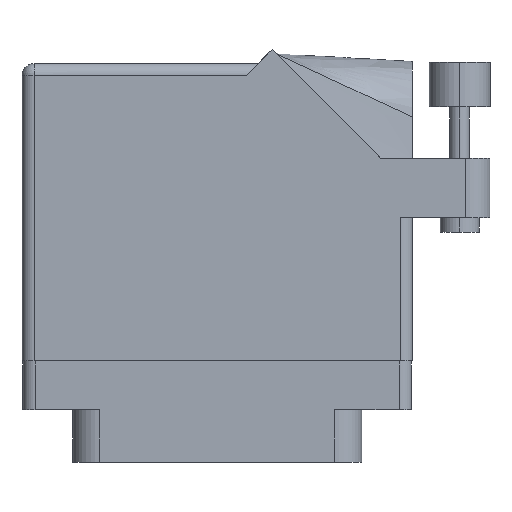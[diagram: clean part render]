
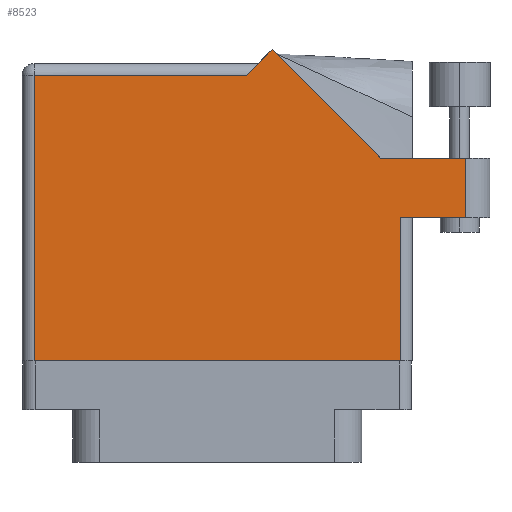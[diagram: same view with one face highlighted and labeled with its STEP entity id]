
A CAD part, front view. The second image highlights one B-rep face of the part: STEP entity #8523.
In plain terms, the highlighted face is planar.
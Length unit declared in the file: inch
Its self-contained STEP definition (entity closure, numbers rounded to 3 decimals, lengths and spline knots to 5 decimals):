
#55 = VECTOR ( 'NONE', #25934, 39.37008 ) ;
#152 = CARTESIAN_POINT ( 'NONE',  ( 0.943, 0.637, 0.455 ) ) ;
#241 = DIRECTION ( 'NONE',  ( 0., 0., -1. ) ) ;
#344 = LINE ( 'NONE', #152, #34561 ) ;
#897 = VECTOR ( 'NONE', #5899, 39.37008 ) ;
#1307 = EDGE_CURVE ( 'NONE', #15576, #29729, #1485, .T. ) ;
#1485 = LINE ( 'NONE', #18802, #12579 ) ;
#2262 = DIRECTION ( 'NONE',  ( -0.707, -0.707, 0. ) ) ;
#2339 = EDGE_CURVE ( 'NONE', #31374, #31788, #14088, .T. ) ;
#3146 = AXIS2_PLACEMENT_3D ( 'NONE', #25574, #241, #20287 ) ;
#3158 = FACE_OUTER_BOUND ( 'NONE', #18967, .T. ) ;
#5257 = VECTOR ( 'NONE', #7692, 39.37008 ) ;
#5899 = DIRECTION ( 'NONE',  ( 1., 0., 0. ) ) ;
#5956 = EDGE_CURVE ( 'NONE', #28163, #32775, #33206, .T. ) ;
#6568 = LINE ( 'NONE', #12225, #14591 ) ;
#6695 = ORIENTED_EDGE ( 'NONE', *, *, #24863, .T. ) ;
#6855 = EDGE_CURVE ( 'NONE', #10171, #27186, #22546, .T. ) ;
#7660 = VECTOR ( 'NONE', #8869, 39.37008 ) ;
#7692 = DIRECTION ( 'NONE',  ( 1., 0., 0. ) ) ;
#8523 = ADVANCED_FACE ( 'NONE', ( #3158 ), #23013, .F. ) ;
#8617 = CARTESIAN_POINT ( 'NONE',  ( 0.943, 0.637, 0.455 ) ) ;
#8869 = DIRECTION ( 'NONE',  ( -1., 0., 0. ) ) ;
#9012 = ORIENTED_EDGE ( 'NONE', *, *, #31876, .T. ) ;
#10103 = LINE ( 'NONE', #24867, #16207 ) ;
#10171 = VERTEX_POINT ( 'NONE', #26170 ) ;
#10815 = VECTOR ( 'NONE', #35545, 39.37008 ) ;
#12225 = CARTESIAN_POINT ( 'NONE',  ( 0.83942, 0.944, 0.455 ) ) ;
#12264 = CARTESIAN_POINT ( 'NONE',  ( -0.943, -0.1, 0.455 ) ) ;
#12579 = VECTOR ( 'NONE', #15686, 39.37008 ) ;
#12587 = ORIENTED_EDGE ( 'NONE', *, *, #17353, .T. ) ;
#13760 = EDGE_CURVE ( 'NONE', #33357, #10171, #10103, .T. ) ;
#14088 = LINE ( 'NONE', #19561, #897 ) ;
#14591 = VECTOR ( 'NONE', #29182, 39.37008 ) ;
#14793 = LINE ( 'NONE', #31575, #55 ) ;
#15576 = VERTEX_POINT ( 'NONE', #21921 ) ;
#15686 = DIRECTION ( 'NONE',  ( -1., 0., 0. ) ) ;
#16207 = VECTOR ( 'NONE', #2262, 39.37008 ) ;
#16347 = CARTESIAN_POINT ( 'NONE',  ( -0.943, 1.368, 0.455 ) ) ;
#17353 = EDGE_CURVE ( 'NONE', #27186, #31374, #24068, .T. ) ;
#18802 = CARTESIAN_POINT ( 'NONE',  ( 1.405, 0.944, 0.455 ) ) ;
#18967 = EDGE_LOOP ( 'NONE', ( #28913, #6695, #33862, #9012, #30236, #19219, #12587, #33225, #22870 ) ) ;
#19219 = ORIENTED_EDGE ( 'NONE', *, *, #6855, .T. ) ;
#19561 = CARTESIAN_POINT ( 'NONE',  ( -1.005, -0.1, 0.455 ) ) ;
#20235 = CARTESIAN_POINT ( 'NONE',  ( 0.28271, 1.50071, 0.455 ) ) ;
#20287 = DIRECTION ( 'NONE',  ( -1., 0., 0. ) ) ;
#21921 = CARTESIAN_POINT ( 'NONE',  ( 1.28, 0.944, 0.455 ) ) ;
#22401 = DIRECTION ( 'NONE',  ( 0., 1., 0. ) ) ;
#22546 = LINE ( 'NONE', #33302, #7660 ) ;
#22817 = CARTESIAN_POINT ( 'NONE',  ( 0.943, -0.1, 0.455 ) ) ;
#22870 = ORIENTED_EDGE ( 'NONE', *, *, #29187, .T. ) ;
#23013 = PLANE ( 'NONE',  #3146 ) ;
#24068 = LINE ( 'NONE', #29710, #10815 ) ;
#24863 = EDGE_CURVE ( 'NONE', #32775, #15576, #14793, .T. ) ;
#24867 = CARTESIAN_POINT ( 'NONE',  ( 0.212, 1.43, 0.455 ) ) ;
#25038 = CARTESIAN_POINT ( 'NONE',  ( 1.28, 0.637, 0.455 ) ) ;
#25574 = CARTESIAN_POINT ( 'NONE',  ( -1.005, 1.43, 0.455 ) ) ;
#25934 = DIRECTION ( 'NONE',  ( 0., 1., 0. ) ) ;
#26170 = CARTESIAN_POINT ( 'NONE',  ( 0.15, 1.368, 0.455 ) ) ;
#27186 = VERTEX_POINT ( 'NONE', #16347 ) ;
#28163 = VERTEX_POINT ( 'NONE', #8617 ) ;
#28913 = ORIENTED_EDGE ( 'NONE', *, *, #5956, .T. ) ;
#29182 = DIRECTION ( 'NONE',  ( -0.707, 0.707, 0. ) ) ;
#29187 = EDGE_CURVE ( 'NONE', #31788, #28163, #344, .T. ) ;
#29710 = CARTESIAN_POINT ( 'NONE',  ( -0.943, -0.1, 0.455 ) ) ;
#29729 = VERTEX_POINT ( 'NONE', #32175 ) ;
#30236 = ORIENTED_EDGE ( 'NONE', *, *, #13760, .T. ) ;
#31374 = VERTEX_POINT ( 'NONE', #12264 ) ;
#31575 = CARTESIAN_POINT ( 'NONE',  ( 1.28, 0.944, 0.455 ) ) ;
#31788 = VERTEX_POINT ( 'NONE', #22817 ) ;
#31876 = EDGE_CURVE ( 'NONE', #29729, #33357, #6568, .T. ) ;
#32175 = CARTESIAN_POINT ( 'NONE',  ( 0.83942, 0.944, 0.455 ) ) ;
#32775 = VERTEX_POINT ( 'NONE', #25038 ) ;
#33206 = LINE ( 'NONE', #35410, #5257 ) ;
#33225 = ORIENTED_EDGE ( 'NONE', *, *, #2339, .T. ) ;
#33302 = CARTESIAN_POINT ( 'NONE',  ( -1.005, 1.368, 0.455 ) ) ;
#33357 = VERTEX_POINT ( 'NONE', #20235 ) ;
#33862 = ORIENTED_EDGE ( 'NONE', *, *, #1307, .T. ) ;
#34561 = VECTOR ( 'NONE', #22401, 39.37008 ) ;
#35410 = CARTESIAN_POINT ( 'NONE',  ( 1.005, 0.637, 0.455 ) ) ;
#35545 = DIRECTION ( 'NONE',  ( 0., -1., 0. ) ) ;
